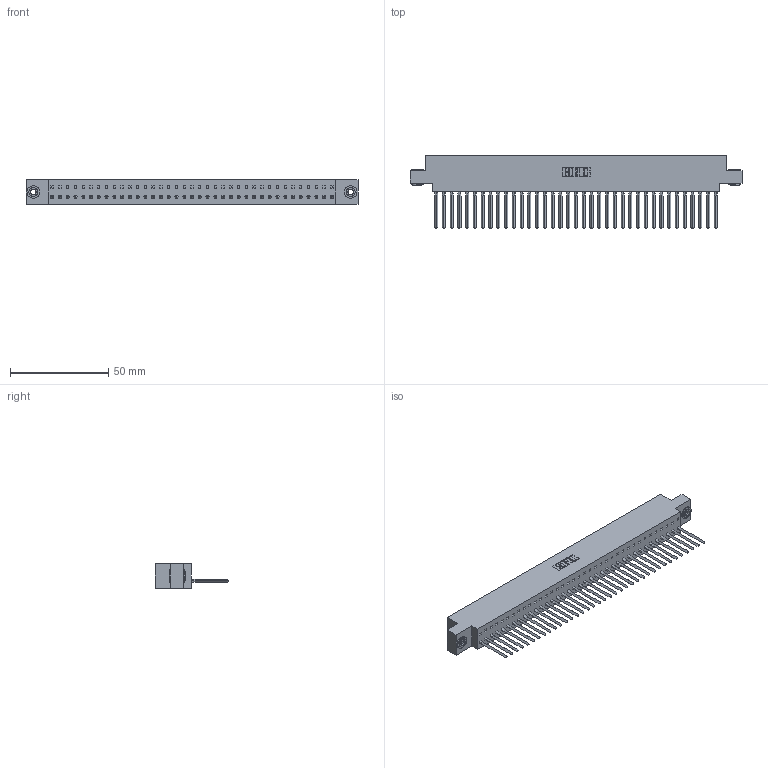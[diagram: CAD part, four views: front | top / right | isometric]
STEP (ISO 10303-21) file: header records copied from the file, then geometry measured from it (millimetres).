
FILE_DESCRIPTION (( 'STEP AP203' ), '1' );
FILE_NAME ('317-037-541-603.STEP', '2020-02-27T23:12:44', ( '' ), ( '' ), 'SwSTEP 2.0', 'SolidWorks 2016', '' );
FILE_SCHEMA (( 'CONFIG_CONTROL_DESIGN' ));
Length unit declared in the file: inch
Products named in the file (4): 317 Part_.156 Dia - TH; 317-037-541-603; 317-290-002_541; 345-250-002_345-250-002-102
Assembly tree (40 placements, depth 2):
  317-037-541-603
    317 Part_.156 Dia - TH
    317-290-002_541  x37
    345-250-002_345-250-002-102  x2
Bounding box: 169.32 x 37.34 x 12.7 mm (x, y, z)
Volume: 27323.1 mm3; surface area: 38657.3 mm2
Topology: 40 solids, 40 shells, 5764 faces, 16409 edges, 10664 vertices
Faces by surface type: plane 4656, cylinder 952, bspline 148, cone 8
Entity records: 55195 total; most frequent: CARTESIAN_POINT 10419, ORIENTED_EDGE 9702, DIRECTION 8007, EDGE_CURVE 4851, LINE 4463, VECTOR 4463, VERTEX_POINT 3224, AXIS2_PLACEMENT_3D 1772
